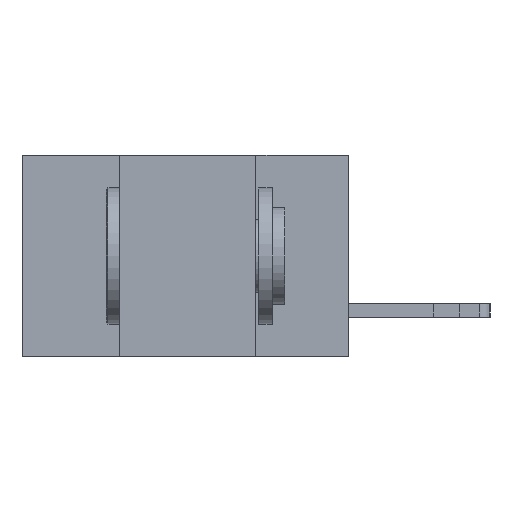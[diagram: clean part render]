
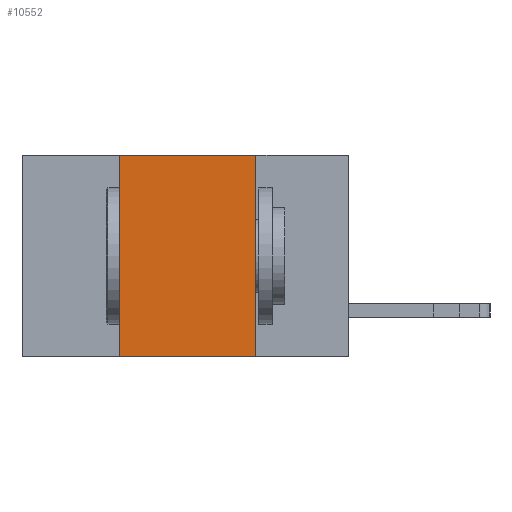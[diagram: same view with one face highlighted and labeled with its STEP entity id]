
A CAD part, left-side view. The second image highlights one B-rep face of the part: STEP entity #10552.
In plain terms, the highlighted planar face has unit normal (-1, 0, 0).
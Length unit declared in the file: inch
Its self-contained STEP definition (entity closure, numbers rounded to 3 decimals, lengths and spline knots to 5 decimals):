
#2488 = DIRECTION ( 'NONE',  ( 0., 0., -1. ) ) ;
#2520 = EDGE_CURVE ( 'NONE', #12411, #14966, #14270, .T. ) ;
#2700 = FACE_OUTER_BOUND ( 'NONE', #15062, .T. ) ;
#2905 = LINE ( 'NONE', #16672, #16341 ) ;
#3160 = EDGE_CURVE ( 'NONE', #12815, #14966, #2905, .T. ) ;
#4367 = DIRECTION ( 'NONE',  ( 0., -1., 0. ) ) ;
#5267 = ORIENTED_EDGE ( 'NONE', *, *, #16518, .F. ) ;
#5514 = CARTESIAN_POINT ( 'NONE',  ( 0., 0.42, -0.37 ) ) ;
#6692 = PLANE ( 'NONE',  #7224 ) ;
#7224 = AXIS2_PLACEMENT_3D ( 'NONE', #16802, #10660, #2488 ) ;
#7460 = DIRECTION ( 'NONE',  ( 0., -1., 0. ) ) ;
#7990 = ORIENTED_EDGE ( 'NONE', *, *, #3160, .T. ) ;
#8591 = VECTOR ( 'NONE', #7460, 39.37008 ) ;
#8898 = ORIENTED_EDGE ( 'NONE', *, *, #10958, .F. ) ;
#10152 = CARTESIAN_POINT ( 'NONE',  ( 0., 0.17, 0. ) ) ;
#10552 = ADVANCED_FACE ( 'NONE', ( #2700 ), #6692, .F. ) ;
#10660 = DIRECTION ( 'NONE',  ( 1., 0., 0. ) ) ;
#10826 = CARTESIAN_POINT ( 'NONE',  ( 0., 0.17, -0.37 ) ) ;
#10958 = EDGE_CURVE ( 'NONE', #14445, #12411, #15252, .T. ) ;
#11444 = CARTESIAN_POINT ( 'NONE',  ( 0., 0.17, 0. ) ) ;
#11689 = DIRECTION ( 'NONE',  ( 0., 0., -1. ) ) ;
#11879 = CARTESIAN_POINT ( 'NONE',  ( 0., 0.42, 0. ) ) ;
#12411 = VERTEX_POINT ( 'NONE', #10152 ) ;
#12520 = CARTESIAN_POINT ( 'NONE',  ( 0., 0.6, 0. ) ) ;
#12815 = VERTEX_POINT ( 'NONE', #5514 ) ;
#13388 = ORIENTED_EDGE ( 'NONE', *, *, #2520, .F. ) ;
#13921 = LINE ( 'NONE', #11879, #16803 ) ;
#14270 = LINE ( 'NONE', #11444, #17128 ) ;
#14399 = DIRECTION ( 'NONE',  ( 0., 0., 1. ) ) ;
#14445 = VERTEX_POINT ( 'NONE', #16396 ) ;
#14966 = VERTEX_POINT ( 'NONE', #10826 ) ;
#15062 = EDGE_LOOP ( 'NONE', ( #13388, #8898, #5267, #7990 ) ) ;
#15252 = LINE ( 'NONE', #12520, #8591 ) ;
#16341 = VECTOR ( 'NONE', #4367, 39.37008 ) ;
#16396 = CARTESIAN_POINT ( 'NONE',  ( 0., 0.42, 0. ) ) ;
#16518 = EDGE_CURVE ( 'NONE', #12815, #14445, #13921, .T. ) ;
#16672 = CARTESIAN_POINT ( 'NONE',  ( 0., 0.6, -0.37 ) ) ;
#16802 = CARTESIAN_POINT ( 'NONE',  ( 0., 0.6, 0. ) ) ;
#16803 = VECTOR ( 'NONE', #14399, 39.37008 ) ;
#17128 = VECTOR ( 'NONE', #11689, 39.37008 ) ;
